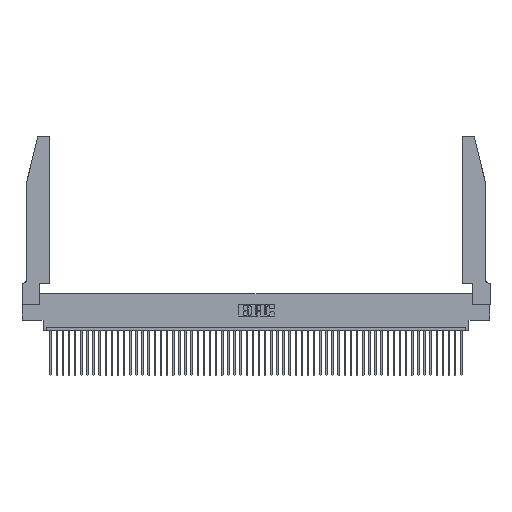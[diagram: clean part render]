
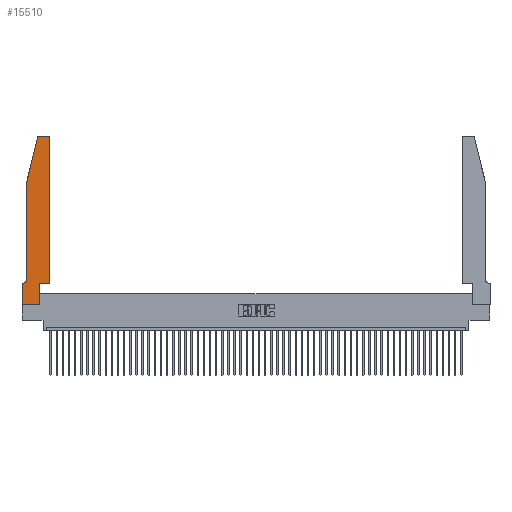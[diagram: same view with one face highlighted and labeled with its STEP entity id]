
A CAD part, top view. The second image highlights one B-rep face of the part: STEP entity #15510.
In plain terms, the highlighted planar face has unit normal (0, 0, 1).
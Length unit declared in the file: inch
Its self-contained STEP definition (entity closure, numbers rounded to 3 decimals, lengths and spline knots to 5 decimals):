
#371 = LINE ( 'NONE', #28497, #49229 ) ;
#652 = VECTOR ( 'NONE', #39920, 39.37008 ) ;
#745 = CARTESIAN_POINT ( 'NONE',  ( 0.0055, 0.35, 0.37 ) ) ;
#877 = VERTEX_POINT ( 'NONE', #24543 ) ;
#1531 = CIRCLE ( 'NONE', #8476, 0.03 ) ;
#3271 = CARTESIAN_POINT ( 'NONE',  ( 0.4505, 2.72, 0.37 ) ) ;
#3282 = VECTOR ( 'NONE', #41407, 39.37008 ) ;
#3642 = EDGE_CURVE ( 'NONE', #50617, #40743, #12221, .T. ) ;
#4525 = CARTESIAN_POINT ( 'NONE',  ( 0.0055, 0.42, 0.37 ) ) ;
#4591 = ORIENTED_EDGE ( 'NONE', *, *, #12596, .T. ) ;
#5165 = LINE ( 'NONE', #18508, #37525 ) ;
#5298 = VERTEX_POINT ( 'NONE', #35198 ) ;
#6599 = CARTESIAN_POINT ( 'NONE',  ( 0.2605, 2.75, 0.37 ) ) ;
#7038 = DIRECTION ( 'NONE',  ( 0., 0., -1. ) ) ;
#8476 = AXIS2_PLACEMENT_3D ( 'NONE', #29281, #9162, #21554 ) ;
#8825 = VECTOR ( 'NONE', #27049, 39.37008 ) ;
#9084 = CARTESIAN_POINT ( 'NONE',  ( 0.4205, 2.72, 0.37 ) ) ;
#9162 = DIRECTION ( 'NONE',  ( 0., 0., 1. ) ) ;
#9288 = CARTESIAN_POINT ( 'NONE',  ( 0., 0., 0.37 ) ) ;
#9331 = VERTEX_POINT ( 'NONE', #3271 ) ;
#10320 = ORIENTED_EDGE ( 'NONE', *, *, #43419, .T. ) ;
#10606 = DIRECTION ( 'NONE',  ( 1., 0., 0. ) ) ;
#10816 = LINE ( 'NONE', #36443, #8825 ) ;
#11146 = ORIENTED_EDGE ( 'NONE', *, *, #18153, .T. ) ;
#11218 = ORIENTED_EDGE ( 'NONE', *, *, #40868, .T. ) ;
#11516 = DIRECTION ( 'NONE',  ( 1., 0., 0. ) ) ;
#12221 = LINE ( 'NONE', #34931, #23033 ) ;
#12596 = EDGE_CURVE ( 'NONE', #45494, #37564, #5165, .T. ) ;
#13768 = AXIS2_PLACEMENT_3D ( 'NONE', #48375, #27902, #11516 ) ;
#13924 = CARTESIAN_POINT ( 'NONE',  ( 0.284, 2.75, 0.37 ) ) ;
#14284 = EDGE_CURVE ( 'NONE', #20727, #45494, #10816, .T. ) ;
#15331 = DIRECTION ( 'NONE',  ( -1., 0., 0. ) ) ;
#15510 = ADVANCED_FACE ( 'NONE', ( #52588 ), #44312, .T. ) ;
#15831 = CARTESIAN_POINT ( 'NONE',  ( 0.0755, 2., 0.37 ) ) ;
#15846 = VECTOR ( 'NONE', #18068, 39.37008 ) ;
#15883 = LINE ( 'NONE', #9288, #3282 ) ;
#16595 = LINE ( 'NONE', #52364, #652 ) ;
#18068 = DIRECTION ( 'NONE',  ( 0., 1., 0. ) ) ;
#18153 = EDGE_CURVE ( 'NONE', #40743, #9331, #25321, .T. ) ;
#18181 = EDGE_CURVE ( 'NONE', #5298, #41179, #36188, .T. ) ;
#18394 = ORIENTED_EDGE ( 'NONE', *, *, #14284, .T. ) ;
#18451 = CARTESIAN_POINT ( 'NONE',  ( 0.2865, 0.35, 0.37 ) ) ;
#18508 = CARTESIAN_POINT ( 'NONE',  ( 0.0755, 2., 0.37 ) ) ;
#19213 = LINE ( 'NONE', #35847, #35082 ) ;
#19421 = ORIENTED_EDGE ( 'NONE', *, *, #47540, .T. ) ;
#20727 = VERTEX_POINT ( 'NONE', #26206 ) ;
#20899 = CARTESIAN_POINT ( 'NONE',  ( 0.2865, 0., 0.37 ) ) ;
#21554 = DIRECTION ( 'NONE',  ( 1., 0., 0. ) ) ;
#21939 = CIRCLE ( 'NONE', #40882, 0.03 ) ;
#22285 = ORIENTED_EDGE ( 'NONE', *, *, #27099, .T. ) ;
#23033 = VECTOR ( 'NONE', #10606, 39.37008 ) ;
#24543 = CARTESIAN_POINT ( 'NONE',  ( 0., 0., 0.37 ) ) ;
#25321 = LINE ( 'NONE', #51103, #15846 ) ;
#26206 = CARTESIAN_POINT ( 'NONE',  ( 0.25487, 2.72718, 0.37 ) ) ;
#26218 = ORIENTED_EDGE ( 'NONE', *, *, #28756, .T. ) ;
#27049 = DIRECTION ( 'NONE',  ( -0.239, -0.971, 0. ) ) ;
#27099 = EDGE_CURVE ( 'NONE', #37564, #29750, #35677, .T. ) ;
#27902 = DIRECTION ( 'NONE',  ( 0., 0., 1. ) ) ;
#28497 = CARTESIAN_POINT ( 'NONE',  ( 0., 0., 0.37 ) ) ;
#28756 = EDGE_CURVE ( 'NONE', #41179, #20727, #1531, .T. ) ;
#28808 = DIRECTION ( 'NONE',  ( 0., -1., 0. ) ) ;
#28836 = CARTESIAN_POINT ( 'NONE',  ( 0., 0.35, 0.37 ) ) ;
#29281 = CARTESIAN_POINT ( 'NONE',  ( 0.284, 2.72, 0.37 ) ) ;
#29552 = ORIENTED_EDGE ( 'NONE', *, *, #33250, .T. ) ;
#29750 = VERTEX_POINT ( 'NONE', #745 ) ;
#30476 = VECTOR ( 'NONE', #15331, 39.37008 ) ;
#30992 = DIRECTION ( 'NONE',  ( 0., -1., 0. ) ) ;
#33088 = VERTEX_POINT ( 'NONE', #28836 ) ;
#33225 = EDGE_CURVE ( 'NONE', #9331, #5298, #21939, .T. ) ;
#33250 = EDGE_CURVE ( 'NONE', #33088, #877, #371, .T. ) ;
#34931 = CARTESIAN_POINT ( 'NONE',  ( 0.4505, 0.35, 0.37 ) ) ;
#35082 = VECTOR ( 'NONE', #52173, 39.37008 ) ;
#35198 = CARTESIAN_POINT ( 'NONE',  ( 0.4205, 2.75, 0.37 ) ) ;
#35677 = CIRCLE ( 'NONE', #50917, 0.07 ) ;
#35847 = CARTESIAN_POINT ( 'NONE',  ( 0.2865, 0.35, 0.37 ) ) ;
#36188 = LINE ( 'NONE', #6599, #30476 ) ;
#36443 = CARTESIAN_POINT ( 'NONE',  ( 0.0755, 2., 0.37 ) ) ;
#37525 = VECTOR ( 'NONE', #30992, 39.37008 ) ;
#37564 = VERTEX_POINT ( 'NONE', #39542 ) ;
#37817 = EDGE_LOOP ( 'NONE', ( #51748, #26218, #18394, #4591, #22285, #11218, #29552, #19421, #10320, #50392, #11146, #43899 ) ) ;
#38194 = DIRECTION ( 'NONE',  ( 1., 0., 0. ) ) ;
#39542 = CARTESIAN_POINT ( 'NONE',  ( 0.0755, 0.42, 0.37 ) ) ;
#39920 = DIRECTION ( 'NONE',  ( -1., 0., 0. ) ) ;
#40743 = VERTEX_POINT ( 'NONE', #46096 ) ;
#40868 = EDGE_CURVE ( 'NONE', #29750, #33088, #16595, .T. ) ;
#40882 = AXIS2_PLACEMENT_3D ( 'NONE', #9084, #42469, #38194 ) ;
#41179 = VERTEX_POINT ( 'NONE', #13924 ) ;
#41407 = DIRECTION ( 'NONE',  ( 1., 0., 0. ) ) ;
#42469 = DIRECTION ( 'NONE',  ( 0., 0., 1. ) ) ;
#43419 = EDGE_CURVE ( 'NONE', #52327, #50617, #19213, .T. ) ;
#43899 = ORIENTED_EDGE ( 'NONE', *, *, #33225, .T. ) ;
#44312 = PLANE ( 'NONE',  #13768 ) ;
#44604 = DIRECTION ( 'NONE',  ( -1., 0., 0. ) ) ;
#45494 = VERTEX_POINT ( 'NONE', #15831 ) ;
#46096 = CARTESIAN_POINT ( 'NONE',  ( 0.4505, 0.35, 0.37 ) ) ;
#47540 = EDGE_CURVE ( 'NONE', #877, #52327, #15883, .T. ) ;
#48375 = CARTESIAN_POINT ( 'NONE',  ( 0., 0.35, 0.37 ) ) ;
#49229 = VECTOR ( 'NONE', #28808, 39.37008 ) ;
#50392 = ORIENTED_EDGE ( 'NONE', *, *, #3642, .T. ) ;
#50617 = VERTEX_POINT ( 'NONE', #18451 ) ;
#50917 = AXIS2_PLACEMENT_3D ( 'NONE', #4525, #7038, #44604 ) ;
#51103 = CARTESIAN_POINT ( 'NONE',  ( 0.4505, 0.35, 0.37 ) ) ;
#51748 = ORIENTED_EDGE ( 'NONE', *, *, #18181, .T. ) ;
#52173 = DIRECTION ( 'NONE',  ( 0., 1., 0. ) ) ;
#52327 = VERTEX_POINT ( 'NONE', #20899 ) ;
#52364 = CARTESIAN_POINT ( 'NONE',  ( 0.0755, 0.35, 0.37 ) ) ;
#52588 = FACE_OUTER_BOUND ( 'NONE', #37817, .T. ) ;
